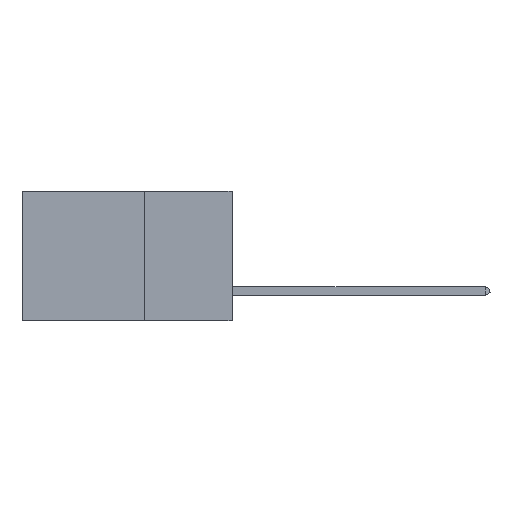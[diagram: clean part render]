
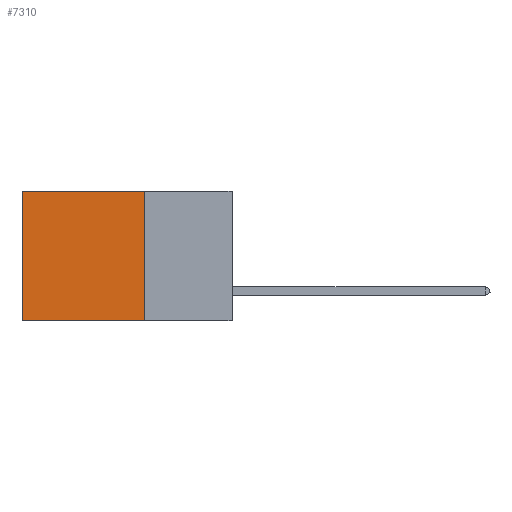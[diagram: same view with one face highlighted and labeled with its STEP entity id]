
A CAD part, left-side view. The second image highlights one B-rep face of the part: STEP entity #7310.
In plain terms, the highlighted planar face has unit normal (-1, 0, 0).
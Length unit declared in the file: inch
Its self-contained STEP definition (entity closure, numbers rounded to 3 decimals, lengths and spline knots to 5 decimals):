
#688 = DIRECTION ( 'NONE',  ( 0., 0., -1. ) ) ;
#1119 = CARTESIAN_POINT ( 'NONE',  ( 0.2875, 0.6, 0. ) ) ;
#1635 = DIRECTION ( 'NONE',  ( 0., 1., 0. ) ) ;
#2121 = LINE ( 'NONE', #11240, #18655 ) ;
#2203 = VERTEX_POINT ( 'NONE', #22242 ) ;
#3431 = VERTEX_POINT ( 'NONE', #1119 ) ;
#3574 = DIRECTION ( 'NONE',  ( 0., 0., -1. ) ) ;
#4256 = DIRECTION ( 'NONE',  ( 0., 1., 0. ) ) ;
#5148 = EDGE_CURVE ( 'NONE', #8836, #3431, #21701, .T. ) ;
#5219 = EDGE_CURVE ( 'NONE', #2203, #20236, #7635, .T. ) ;
#6081 = CARTESIAN_POINT ( 'NONE',  ( 0.2875, 0.25, 0. ) ) ;
#6133 = VECTOR ( 'NONE', #3574, 39.37008 ) ;
#6419 = PLANE ( 'NONE',  #6616 ) ;
#6616 = AXIS2_PLACEMENT_3D ( 'NONE', #14995, #18716, #18797 ) ;
#7077 = VECTOR ( 'NONE', #1635, 39.37008 ) ;
#7310 = ADVANCED_FACE ( 'NONE', ( #11016 ), #6419, .F. ) ;
#7635 = LINE ( 'NONE', #19195, #7077 ) ;
#8836 = VERTEX_POINT ( 'NONE', #22280 ) ;
#9607 = EDGE_CURVE ( 'NONE', #3431, #20236, #2121, .T. ) ;
#11016 = FACE_OUTER_BOUND ( 'NONE', #14566, .T. ) ;
#11240 = CARTESIAN_POINT ( 'NONE',  ( 0.2875, 0.6, 0. ) ) ;
#12010 = LINE ( 'NONE', #12389, #6133 ) ;
#12150 = ORIENTED_EDGE ( 'NONE', *, *, #9607, .T. ) ;
#12389 = CARTESIAN_POINT ( 'NONE',  ( 0.2875, 0.25, 0. ) ) ;
#12961 = ORIENTED_EDGE ( 'NONE', *, *, #5148, .T. ) ;
#14254 = ORIENTED_EDGE ( 'NONE', *, *, #5219, .F. ) ;
#14566 = EDGE_LOOP ( 'NONE', ( #12150, #14254, #21644, #12961 ) ) ;
#14995 = CARTESIAN_POINT ( 'NONE',  ( 0.2875, 0.25, 0. ) ) ;
#17956 = CARTESIAN_POINT ( 'NONE',  ( 0.2875, 0.6, -0.37 ) ) ;
#18655 = VECTOR ( 'NONE', #688, 39.37008 ) ;
#18716 = DIRECTION ( 'NONE',  ( 1., 0., 0. ) ) ;
#18797 = DIRECTION ( 'NONE',  ( 0., 0., -1. ) ) ;
#19195 = CARTESIAN_POINT ( 'NONE',  ( 0.2875, 0.25, -0.37 ) ) ;
#20236 = VERTEX_POINT ( 'NONE', #17956 ) ;
#20887 = VECTOR ( 'NONE', #4256, 39.37008 ) ;
#21644 = ORIENTED_EDGE ( 'NONE', *, *, #21826, .F. ) ;
#21701 = LINE ( 'NONE', #6081, #20887 ) ;
#21826 = EDGE_CURVE ( 'NONE', #8836, #2203, #12010, .T. ) ;
#22242 = CARTESIAN_POINT ( 'NONE',  ( 0.2875, 0.25, -0.37 ) ) ;
#22280 = CARTESIAN_POINT ( 'NONE',  ( 0.2875, 0.25, 0. ) ) ;
